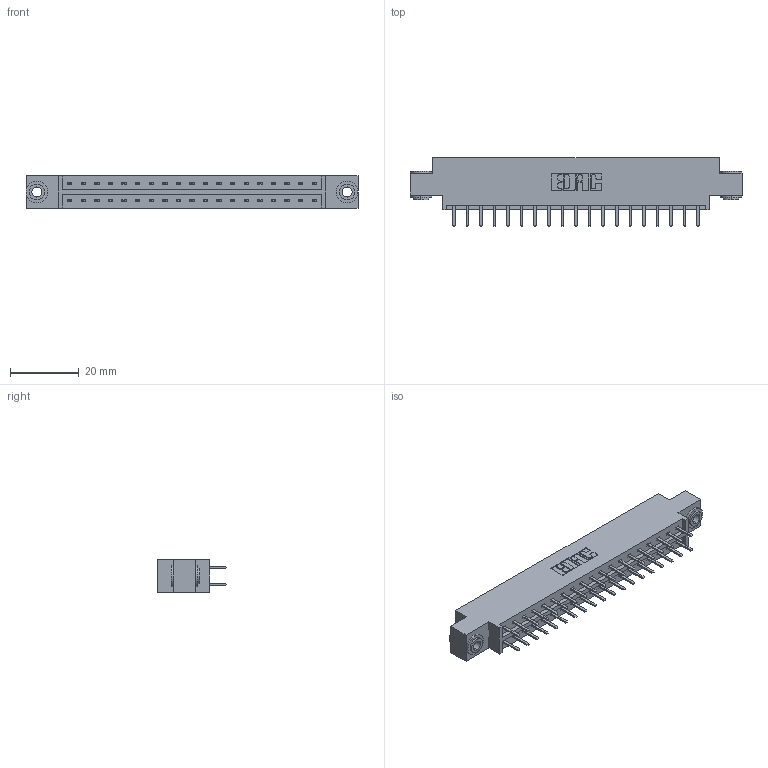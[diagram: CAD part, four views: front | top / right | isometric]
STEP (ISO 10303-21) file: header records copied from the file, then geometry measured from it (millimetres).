
FILE_DESCRIPTION (( 'STEP AP203' ), '1' );
FILE_NAME ('833-038-520-803.STEP', '2020-06-03T06:28:44', ( '' ), ( '' ), 'SwSTEP 2.0', 'SolidWorks 2020', '' );
FILE_SCHEMA (( 'CONFIG_CONTROL_DESIGN' ));
Length unit declared in the file: inch
Products named in the file (4): 833 Part_Offset - .156 Dia - TH; 345-250-002_345-250-002-102; 833-038-520-803; 345-292-001_345-293-120
Assembly tree (41 placements, depth 2):
  833-038-520-803
    833 Part_Offset - .156 Dia - TH
    345-292-001_345-293-120  x38
    345-250-002_345-250-002-102  x2
Bounding box: 96.82 x 20.02 x 9.4 mm (x, y, z)
Volume: 9445.1 mm3; surface area: 11316.7 mm2
Topology: 41 solids, 41 shells, 2284 faces, 6593 edges, 4290 vertices
Faces by surface type: plane 1528, cylinder 748, cone 8
Entity records: 16094 total; most frequent: CARTESIAN_POINT 2685, ORIENTED_EDGE 2602, DIRECTION 2355, EDGE_CURVE 1301, VECTOR 1145, LINE 1145, VERTEX_POINT 862, AXIS2_PLACEMENT_3D 605
